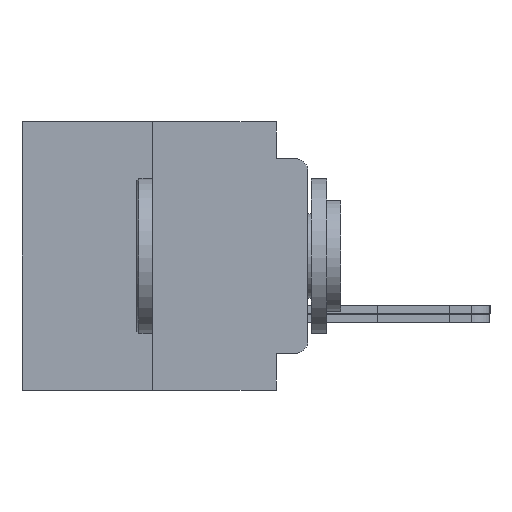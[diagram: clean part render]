
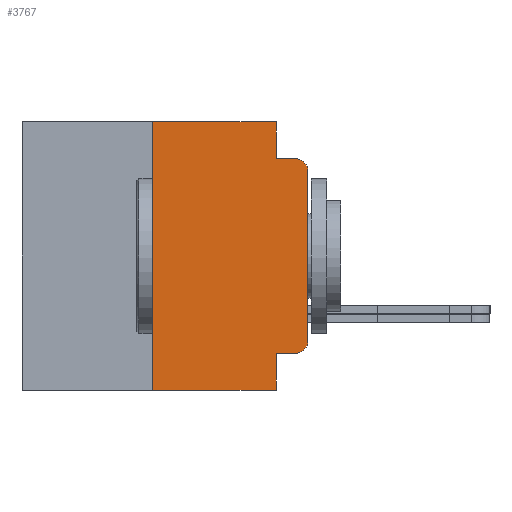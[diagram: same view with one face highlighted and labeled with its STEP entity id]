
A CAD part, left-side view. The second image highlights one B-rep face of the part: STEP entity #3767.
In plain terms, the highlighted planar face has unit normal (-1, 0, 0).
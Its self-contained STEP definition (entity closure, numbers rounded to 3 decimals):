
#11 = ORIENTED_EDGE ( 'NONE', *, *, #1077, .T. ) ;
#706 = LINE ( 'NONE', #26699, #23517 ) ;
#740 = DIRECTION ( 'NONE',  ( 0., 0., -1. ) ) ;
#1066 = VECTOR ( 'NONE', #28178, 1000. ) ;
#1077 = EDGE_CURVE ( 'NONE', #12078, #27395, #22606, .T. ) ;
#1979 = VERTEX_POINT ( 'NONE', #10958 ) ;
#3383 = CIRCLE ( 'NONE', #23823, 0.508 ) ;
#3448 = VERTEX_POINT ( 'NONE', #13968 ) ;
#3667 = VECTOR ( 'NONE', #12365, 1000. ) ;
#3701 = CARTESIAN_POINT ( 'NONE',  ( -75.603, 1.295, -3.975 ) ) ;
#3767 = ADVANCED_FACE ( 'NONE', ( #5107 ), #13548, .F. ) ;
#4213 = CARTESIAN_POINT ( 'NONE',  ( -75.603, 0., -3.467 ) ) ;
#4759 = EDGE_CURVE ( 'NONE', #10068, #3448, #20568, .T. ) ;
#4928 = CARTESIAN_POINT ( 'NONE',  ( -75.603, 0.508, 3.467 ) ) ;
#4961 = VERTEX_POINT ( 'NONE', #4213 ) ;
#5107 = FACE_OUTER_BOUND ( 'NONE', #25506, .T. ) ;
#5617 = VECTOR ( 'NONE', #22344, 1000. ) ;
#5634 = ORIENTED_EDGE ( 'NONE', *, *, #25230, .F. ) ;
#5847 = DIRECTION ( 'NONE',  ( 0., -1., 0. ) ) ;
#5990 = CARTESIAN_POINT ( 'NONE',  ( -75.603, 6.35, -5.486 ) ) ;
#6585 = EDGE_CURVE ( 'NONE', #18890, #1979, #13603, .T. ) ;
#7333 = CARTESIAN_POINT ( 'NONE',  ( -75.603, 6.35, 5.486 ) ) ;
#7933 = DIRECTION ( 'NONE',  ( 0., 0., 1. ) ) ;
#8129 = DIRECTION ( 'NONE',  ( 0., 0., -1. ) ) ;
#8734 = AXIS2_PLACEMENT_3D ( 'NONE', #4928, #13733, #22678 ) ;
#8773 = EDGE_CURVE ( 'NONE', #3448, #26976, #10885, .T. ) ;
#9017 = DIRECTION ( 'NONE',  ( 1., 0., 0. ) ) ;
#10006 = CARTESIAN_POINT ( 'NONE',  ( -75.603, 1.295, -3.975 ) ) ;
#10068 = VERTEX_POINT ( 'NONE', #7333 ) ;
#10848 = VERTEX_POINT ( 'NONE', #25891 ) ;
#10885 = LINE ( 'NONE', #28518, #14306 ) ;
#10887 = CARTESIAN_POINT ( 'NONE',  ( -75.603, 6.35, -5.486 ) ) ;
#10958 = CARTESIAN_POINT ( 'NONE',  ( -75.603, 0.508, 3.975 ) ) ;
#11143 = VECTOR ( 'NONE', #26238, 1000. ) ;
#11883 = CARTESIAN_POINT ( 'NONE',  ( -75.603, 1.295, 3.975 ) ) ;
#12078 = VERTEX_POINT ( 'NONE', #10006 ) ;
#12167 = LINE ( 'NONE', #5990, #26625 ) ;
#12292 = CARTESIAN_POINT ( 'NONE',  ( -75.603, 1.295, 3.975 ) ) ;
#12365 = DIRECTION ( 'NONE',  ( 0., -1., 0. ) ) ;
#13428 = ORIENTED_EDGE ( 'NONE', *, *, #4759, .F. ) ;
#13548 = PLANE ( 'NONE',  #14795 ) ;
#13603 = CIRCLE ( 'NONE', #8734, 0.508 ) ;
#13733 = DIRECTION ( 'NONE',  ( -1., 0., 0. ) ) ;
#13968 = CARTESIAN_POINT ( 'NONE',  ( -75.603, 1.295, 5.486 ) ) ;
#14306 = VECTOR ( 'NONE', #740, 1000. ) ;
#14795 = AXIS2_PLACEMENT_3D ( 'NONE', #15769, #9017, #26650 ) ;
#15550 = ORIENTED_EDGE ( 'NONE', *, *, #6585, .T. ) ;
#15769 = CARTESIAN_POINT ( 'NONE',  ( -75.603, 11.684, 5.486 ) ) ;
#15815 = DIRECTION ( 'NONE',  ( 0., -1., 0. ) ) ;
#15983 = LINE ( 'NONE', #22241, #5617 ) ;
#16286 = VERTEX_POINT ( 'NONE', #10887 ) ;
#16673 = ORIENTED_EDGE ( 'NONE', *, *, #25294, .F. ) ;
#16756 = EDGE_CURVE ( 'NONE', #27395, #4961, #3383, .T. ) ;
#16994 = LINE ( 'NONE', #12292, #1066 ) ;
#17100 = CARTESIAN_POINT ( 'NONE',  ( -75.603, 0.508, -3.467 ) ) ;
#17790 = CARTESIAN_POINT ( 'NONE',  ( -75.603, 0.508, -3.975 ) ) ;
#18173 = ORIENTED_EDGE ( 'NONE', *, *, #8773, .F. ) ;
#18827 = VECTOR ( 'NONE', #5847, 1000. ) ;
#18890 = VERTEX_POINT ( 'NONE', #27622 ) ;
#19200 = ORIENTED_EDGE ( 'NONE', *, *, #26910, .T. ) ;
#19290 = DIRECTION ( 'NONE',  ( -1., 0., 0. ) ) ;
#19840 = EDGE_CURVE ( 'NONE', #4961, #18890, #15983, .T. ) ;
#20568 = LINE ( 'NONE', #20912, #3667 ) ;
#20912 = CARTESIAN_POINT ( 'NONE',  ( -75.603, 11.684, 5.486 ) ) ;
#21423 = CARTESIAN_POINT ( 'NONE',  ( -75.603, 1.295, 0. ) ) ;
#22241 = CARTESIAN_POINT ( 'NONE',  ( -75.603, 0., 5.486 ) ) ;
#22344 = DIRECTION ( 'NONE',  ( 0., 0., 1. ) ) ;
#22366 = ORIENTED_EDGE ( 'NONE', *, *, #16756, .T. ) ;
#22606 = LINE ( 'NONE', #3701, #18827 ) ;
#22678 = DIRECTION ( 'NONE',  ( 0., 0., -1. ) ) ;
#23517 = VECTOR ( 'NONE', #15815, 1000. ) ;
#23823 = AXIS2_PLACEMENT_3D ( 'NONE', #17100, #19290, #8129 ) ;
#25230 = EDGE_CURVE ( 'NONE', #26976, #1979, #16994, .T. ) ;
#25294 = EDGE_CURVE ( 'NONE', #16286, #10068, #12167, .T. ) ;
#25320 = EDGE_CURVE ( 'NONE', #12078, #10848, #25608, .T. ) ;
#25506 = EDGE_LOOP ( 'NONE', ( #11, #22366, #25603, #15550, #5634, #18173, #13428, #16673, #19200, #27184 ) ) ;
#25603 = ORIENTED_EDGE ( 'NONE', *, *, #19840, .T. ) ;
#25608 = LINE ( 'NONE', #21423, #11143 ) ;
#25891 = CARTESIAN_POINT ( 'NONE',  ( -75.603, 1.295, -5.486 ) ) ;
#26238 = DIRECTION ( 'NONE',  ( 0., 0., -1. ) ) ;
#26625 = VECTOR ( 'NONE', #7933, 1000. ) ;
#26650 = DIRECTION ( 'NONE',  ( 0., 0., -1. ) ) ;
#26699 = CARTESIAN_POINT ( 'NONE',  ( -75.603, 11.684, -5.486 ) ) ;
#26910 = EDGE_CURVE ( 'NONE', #16286, #10848, #706, .T. ) ;
#26976 = VERTEX_POINT ( 'NONE', #11883 ) ;
#27184 = ORIENTED_EDGE ( 'NONE', *, *, #25320, .F. ) ;
#27395 = VERTEX_POINT ( 'NONE', #17790 ) ;
#27622 = CARTESIAN_POINT ( 'NONE',  ( -75.603, 0., 3.467 ) ) ;
#28178 = DIRECTION ( 'NONE',  ( 0., -1., 0. ) ) ;
#28518 = CARTESIAN_POINT ( 'NONE',  ( -75.603, 1.295, 0. ) ) ;
